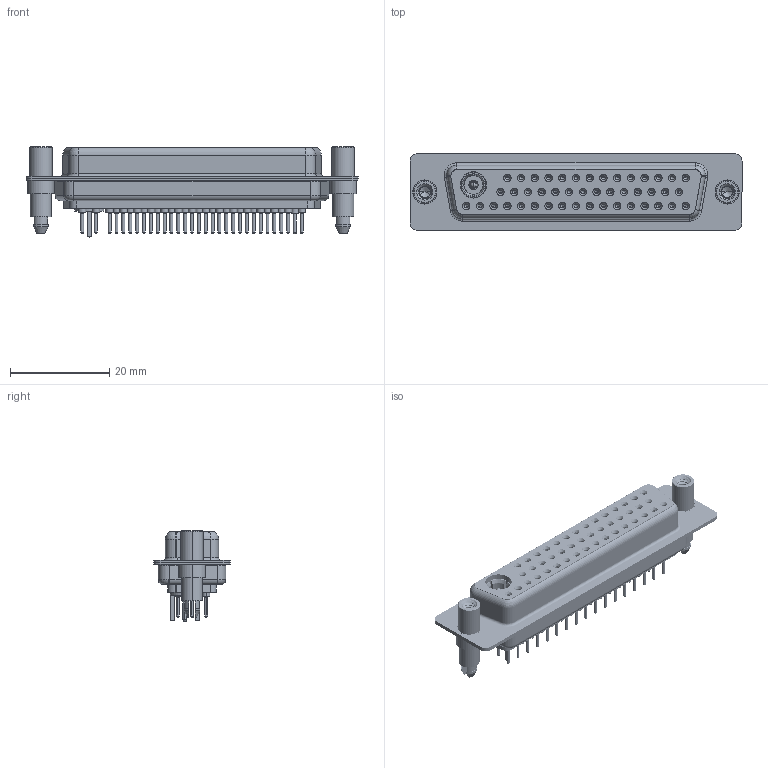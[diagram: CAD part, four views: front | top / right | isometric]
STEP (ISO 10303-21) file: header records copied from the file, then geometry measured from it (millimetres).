
FILE_DESCRIPTION (( 'STEP AP203' ), '1' );
FILE_NAME ('628-47W1624-7T6.STEP', '2019-06-27T03:40:39', ( '' ), ( '' ), 'SwSTEP 2.0', 'SolidWorks 2016', '' );
FILE_SCHEMA (( 'CONFIG_CONTROL_DESIGN' ));
Length unit declared in the file: millimetre
Products named in the file (13): Co-Ax Plug Assy_St; 628Combo Contact Row 2_24; 628Combo Shell Front_50 Contacts; 628Combo Housing_47W1; 628Combo Contact Row 1_24; Pin_Str; Co-Ax Plug_Straight PC Tail; Locking Collar; 628Combo Threaded Standoff and Boardlock_6; Insulator Pin_Straight PC Tail; 628Combo Contact Row 3_24; 628Combo Shell Rear_50 Contacts; 628-47W1624-7T6
Assembly tree (56 placements, depth 3):
  628-47W1624-7T6
    628Combo Housing_47W1
    628Combo Shell Front_50 Contacts
    628Combo Shell Rear_50 Contacts
    628Combo Threaded Standoff and Boardlock_6  x2
    628Combo Contact Row 1_24  x15
    628Combo Contact Row 2_24  x14
    628Combo Contact Row 3_24  x17
    Co-Ax Plug Assy_St
      Co-Ax Plug_Straight PC Tail
      Insulator Pin_Straight PC Tail
      Pin_Str
      Locking Collar
Bounding box: 67 x 15.4 x 18.35 mm (x, y, z)
Volume: 7383.1 mm3; surface area: 15347.5 mm2
Topology: 55 solids, 55 shells, 2975 faces, 6886 edges, 4227 vertices
Faces by surface type: cylinder 1076, plane 829, torus 705, cone 353, bspline 8, sphere 4
Entity records: 35725 total; most frequent: CARTESIAN_POINT 6835, DIRECTION 6126, ORIENTED_EDGE 5026, AXIS2_PLACEMENT_3D 2586, EDGE_CURVE 2513, VERTEX_POINT 1597, CIRCLE 1421, EDGE_LOOP 1390
